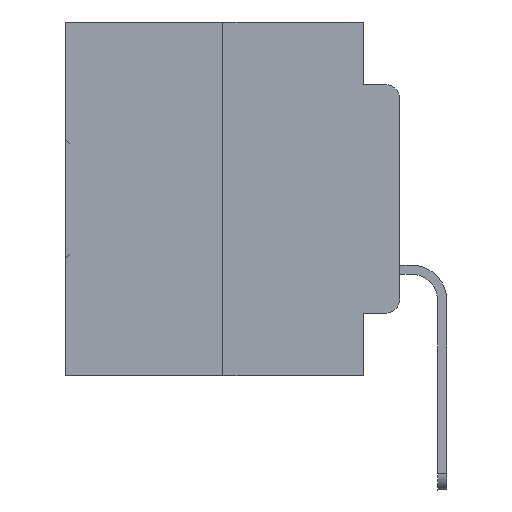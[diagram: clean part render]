
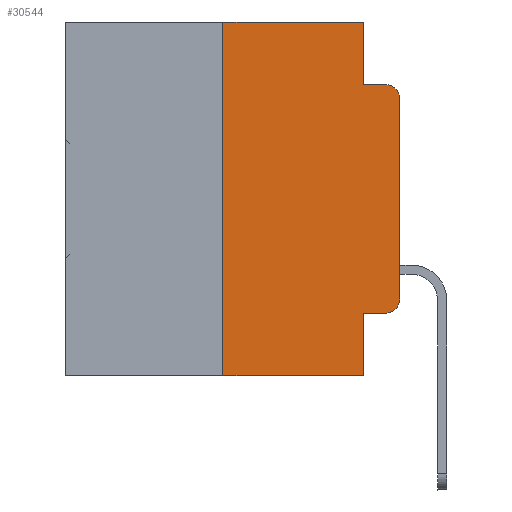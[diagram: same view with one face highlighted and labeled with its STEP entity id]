
A CAD part, left-side view. The second image highlights one B-rep face of the part: STEP entity #30544.
In plain terms, the highlighted planar face has unit normal (-1, 0, 0).
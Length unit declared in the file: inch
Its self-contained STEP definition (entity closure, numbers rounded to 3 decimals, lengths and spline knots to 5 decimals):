
#52 = VERTEX_POINT ( 'NONE', #13875 ) ;
#478 = LINE ( 'NONE', #27303, #2805 ) ;
#544 = CARTESIAN_POINT ( 'NONE',  ( 0., 0.051, -0.0885 ) ) ;
#1140 = LINE ( 'NONE', #4509, #18964 ) ;
#2259 = DIRECTION ( 'NONE',  ( -1., 0., 0. ) ) ;
#2794 = CARTESIAN_POINT ( 'NONE',  ( 0., 0.473, -0.5 ) ) ;
#2805 = VECTOR ( 'NONE', #22407, 39.37008 ) ;
#3796 = CARTESIAN_POINT ( 'NONE',  ( 0., 0.051, 0. ) ) ;
#4190 = EDGE_CURVE ( 'NONE', #5416, #52, #478, .T. ) ;
#4509 = CARTESIAN_POINT ( 'NONE',  ( 0., 0.051, 0. ) ) ;
#4520 = VERTEX_POINT ( 'NONE', #16207 ) ;
#5013 = ORIENTED_EDGE ( 'NONE', *, *, #8382, .T. ) ;
#5364 = DIRECTION ( 'NONE',  ( 1., 0., 0. ) ) ;
#5416 = VERTEX_POINT ( 'NONE', #22446 ) ;
#5852 = LINE ( 'NONE', #2794, #12240 ) ;
#6191 = DIRECTION ( 'NONE',  ( 0., 0., -1. ) ) ;
#6968 = EDGE_CURVE ( 'NONE', #27175, #4520, #15947, .T. ) ;
#8017 = EDGE_CURVE ( 'NONE', #29468, #30045, #26065, .T. ) ;
#8212 = VECTOR ( 'NONE', #13720, 39.37008 ) ;
#8307 = DIRECTION ( 'NONE',  ( 0., -1., 0. ) ) ;
#8382 = EDGE_CURVE ( 'NONE', #4520, #28746, #11686, .T. ) ;
#9094 = ORIENTED_EDGE ( 'NONE', *, *, #10090, .F. ) ;
#9112 = CARTESIAN_POINT ( 'NONE',  ( 0., 0.02, -0.3915 ) ) ;
#9263 = DIRECTION ( 'NONE',  ( 0., 0., 1. ) ) ;
#9894 = ORIENTED_EDGE ( 'NONE', *, *, #8017, .F. ) ;
#9976 = ORIENTED_EDGE ( 'NONE', *, *, #22743, .F. ) ;
#10090 = EDGE_CURVE ( 'NONE', #52, #29468, #15764, .T. ) ;
#10598 = ORIENTED_EDGE ( 'NONE', *, *, #24868, .F. ) ;
#10636 = VECTOR ( 'NONE', #14510, 39.37008 ) ;
#11120 = CARTESIAN_POINT ( 'NONE',  ( 0., 0.02, -0.0885 ) ) ;
#11686 = LINE ( 'NONE', #16403, #30532 ) ;
#11742 = LINE ( 'NONE', #31569, #10636 ) ;
#11845 = VERTEX_POINT ( 'NONE', #20595 ) ;
#11926 = VECTOR ( 'NONE', #23100, 39.37008 ) ;
#12240 = VECTOR ( 'NONE', #22942, 39.37008 ) ;
#13030 = CARTESIAN_POINT ( 'NONE',  ( 0., 0.051, -0.4115 ) ) ;
#13714 = VERTEX_POINT ( 'NONE', #11120 ) ;
#13720 = DIRECTION ( 'NONE',  ( 0., 0., -1. ) ) ;
#13875 = CARTESIAN_POINT ( 'NONE',  ( 0., 0.25, 0. ) ) ;
#14510 = DIRECTION ( 'NONE',  ( 0., -1., 0. ) ) ;
#14910 = VECTOR ( 'NONE', #8307, 39.37008 ) ;
#15287 = DIRECTION ( 'NONE',  ( 0., 0., -1. ) ) ;
#15764 = LINE ( 'NONE', #25997, #14910 ) ;
#15947 = CIRCLE ( 'NONE', #23706, 0.02 ) ;
#16207 = CARTESIAN_POINT ( 'NONE',  ( 0., 0., -0.3915 ) ) ;
#16403 = CARTESIAN_POINT ( 'NONE',  ( 0., 0., 0. ) ) ;
#17199 = ORIENTED_EDGE ( 'NONE', *, *, #4190, .F. ) ;
#18083 = EDGE_LOOP ( 'NONE', ( #5013, #20684, #9976, #9894, #9094, #17199, #26574, #10598, #22253, #24231 ) ) ;
#18100 = EDGE_CURVE ( 'NONE', #19901, #27175, #23259, .T. ) ;
#18621 = AXIS2_PLACEMENT_3D ( 'NONE', #30079, #5364, #15287 ) ;
#18964 = VECTOR ( 'NONE', #19292, 39.37008 ) ;
#19019 = DIRECTION ( 'NONE',  ( -1., 0., 0. ) ) ;
#19024 = CARTESIAN_POINT ( 'NONE',  ( 0., 0.02, -0.4115 ) ) ;
#19292 = DIRECTION ( 'NONE',  ( 0., 0., -1. ) ) ;
#19693 = PLANE ( 'NONE',  #18621 ) ;
#19901 = VERTEX_POINT ( 'NONE', #20212 ) ;
#20173 = FACE_OUTER_BOUND ( 'NONE', #18083, .T. ) ;
#20212 = CARTESIAN_POINT ( 'NONE',  ( 0., 0.051, -0.4115 ) ) ;
#20595 = CARTESIAN_POINT ( 'NONE',  ( 0., 0.051, -0.5 ) ) ;
#20684 = ORIENTED_EDGE ( 'NONE', *, *, #30905, .T. ) ;
#21553 = CARTESIAN_POINT ( 'NONE',  ( 0., 0.051, 0. ) ) ;
#22253 = ORIENTED_EDGE ( 'NONE', *, *, #18100, .T. ) ;
#22407 = DIRECTION ( 'NONE',  ( 0., 0., 1. ) ) ;
#22446 = CARTESIAN_POINT ( 'NONE',  ( 0., 0.25, -0.5 ) ) ;
#22743 = EDGE_CURVE ( 'NONE', #30045, #13714, #11742, .T. ) ;
#22942 = DIRECTION ( 'NONE',  ( 0., -1., 0. ) ) ;
#23100 = DIRECTION ( 'NONE',  ( 0., -1., 0. ) ) ;
#23259 = LINE ( 'NONE', #13030, #11926 ) ;
#23706 = AXIS2_PLACEMENT_3D ( 'NONE', #9112, #19019, #6191 ) ;
#24231 = ORIENTED_EDGE ( 'NONE', *, *, #6968, .T. ) ;
#24357 = CIRCLE ( 'NONE', #29551, 0.02 ) ;
#24868 = EDGE_CURVE ( 'NONE', #19901, #11845, #1140, .T. ) ;
#25997 = CARTESIAN_POINT ( 'NONE',  ( 0., 0.473, 0. ) ) ;
#26065 = LINE ( 'NONE', #3796, #8212 ) ;
#26574 = ORIENTED_EDGE ( 'NONE', *, *, #27088, .T. ) ;
#27088 = EDGE_CURVE ( 'NONE', #5416, #11845, #5852, .T. ) ;
#27133 = CARTESIAN_POINT ( 'NONE',  ( 0., 0.02, -0.1085 ) ) ;
#27175 = VERTEX_POINT ( 'NONE', #19024 ) ;
#27303 = CARTESIAN_POINT ( 'NONE',  ( 0., 0.25, 0. ) ) ;
#28746 = VERTEX_POINT ( 'NONE', #29958 ) ;
#29468 = VERTEX_POINT ( 'NONE', #21553 ) ;
#29551 = AXIS2_PLACEMENT_3D ( 'NONE', #27133, #2259, #29716 ) ;
#29716 = DIRECTION ( 'NONE',  ( 0., 0., -1. ) ) ;
#29958 = CARTESIAN_POINT ( 'NONE',  ( 0., 0., -0.1085 ) ) ;
#30045 = VERTEX_POINT ( 'NONE', #544 ) ;
#30079 = CARTESIAN_POINT ( 'NONE',  ( 0., 0.473, 0. ) ) ;
#30532 = VECTOR ( 'NONE', #9263, 39.37008 ) ;
#30544 = ADVANCED_FACE ( 'NONE', ( #20173 ), #19693, .F. ) ;
#30905 = EDGE_CURVE ( 'NONE', #28746, #13714, #24357, .T. ) ;
#31569 = CARTESIAN_POINT ( 'NONE',  ( 0., 0.051, -0.0885 ) ) ;
